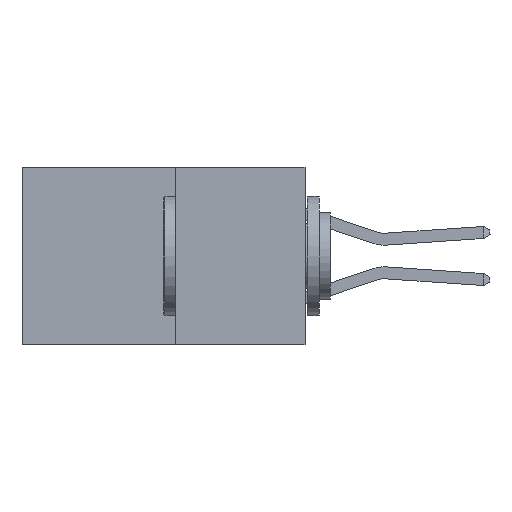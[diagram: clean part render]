
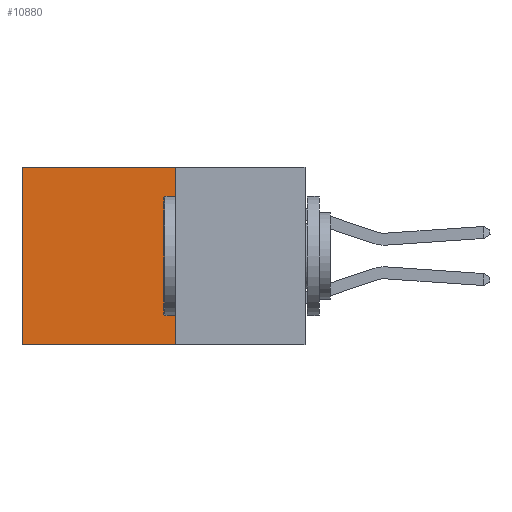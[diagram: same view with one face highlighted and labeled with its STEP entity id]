
A CAD part, left-side view. The second image highlights one B-rep face of the part: STEP entity #10880.
In plain terms, the highlighted planar face has unit normal (-1, 0, 0).
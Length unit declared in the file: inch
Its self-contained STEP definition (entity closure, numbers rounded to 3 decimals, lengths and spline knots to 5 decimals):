
#140 = LINE ( 'NONE', #5915, #18632 ) ;
#176 = VERTEX_POINT ( 'NONE', #14091 ) ;
#646 = DIRECTION ( 'NONE',  ( 0., 0., -1. ) ) ;
#669 = CARTESIAN_POINT ( 'NONE',  ( 0.277, 0.27, -0.37 ) ) ;
#1237 = CARTESIAN_POINT ( 'NONE',  ( 0.277, 0.59, 0. ) ) ;
#1791 = CARTESIAN_POINT ( 'NONE',  ( 0.277, 0.27, -0.37 ) ) ;
#2891 = EDGE_CURVE ( 'NONE', #17351, #176, #18229, .T. ) ;
#3933 = VERTEX_POINT ( 'NONE', #12516 ) ;
#4339 = ORIENTED_EDGE ( 'NONE', *, *, #2891, .F. ) ;
#4376 = LINE ( 'NONE', #13603, #11970 ) ;
#5149 = DIRECTION ( 'NONE',  ( 0., 0., -1. ) ) ;
#5214 = DIRECTION ( 'NONE',  ( 1., 0., 0. ) ) ;
#5915 = CARTESIAN_POINT ( 'NONE',  ( 0.277, 0.27, -0.37 ) ) ;
#8257 = VECTOR ( 'NONE', #16330, 39.37008 ) ;
#10320 = VECTOR ( 'NONE', #646, 39.37008 ) ;
#10880 = ADVANCED_FACE ( 'NONE', ( #18521 ), #13978, .F. ) ;
#11156 = ORIENTED_EDGE ( 'NONE', *, *, #17904, .F. ) ;
#11663 = CARTESIAN_POINT ( 'NONE',  ( 0.277, 0.27, 0. ) ) ;
#11970 = VECTOR ( 'NONE', #14048, 39.37008 ) ;
#12003 = EDGE_CURVE ( 'NONE', #13585, #3933, #4376, .T. ) ;
#12516 = CARTESIAN_POINT ( 'NONE',  ( 0.277, 0.59, -0.37 ) ) ;
#12759 = ORIENTED_EDGE ( 'NONE', *, *, #14764, .T. ) ;
#13585 = VERTEX_POINT ( 'NONE', #1237 ) ;
#13603 = CARTESIAN_POINT ( 'NONE',  ( 0.277, 0.59, -0.37 ) ) ;
#13978 = PLANE ( 'NONE',  #16136 ) ;
#14048 = DIRECTION ( 'NONE',  ( 0., 0., -1. ) ) ;
#14091 = CARTESIAN_POINT ( 'NONE',  ( 0.277, 0.27, -0.37 ) ) ;
#14764 = EDGE_CURVE ( 'NONE', #17351, #13585, #16007, .T. ) ;
#16007 = LINE ( 'NONE', #16311, #8257 ) ;
#16136 = AXIS2_PLACEMENT_3D ( 'NONE', #1791, #5214, #5149 ) ;
#16311 = CARTESIAN_POINT ( 'NONE',  ( 0.277, 0.27, 0. ) ) ;
#16330 = DIRECTION ( 'NONE',  ( 0., 1., 0. ) ) ;
#16653 = ORIENTED_EDGE ( 'NONE', *, *, #12003, .T. ) ;
#17005 = EDGE_LOOP ( 'NONE', ( #16653, #11156, #4339, #12759 ) ) ;
#17351 = VERTEX_POINT ( 'NONE', #11663 ) ;
#17495 = DIRECTION ( 'NONE',  ( 0., 1., 0. ) ) ;
#17904 = EDGE_CURVE ( 'NONE', #176, #3933, #140, .T. ) ;
#18229 = LINE ( 'NONE', #669, #10320 ) ;
#18521 = FACE_OUTER_BOUND ( 'NONE', #17005, .T. ) ;
#18632 = VECTOR ( 'NONE', #17495, 39.37008 ) ;
